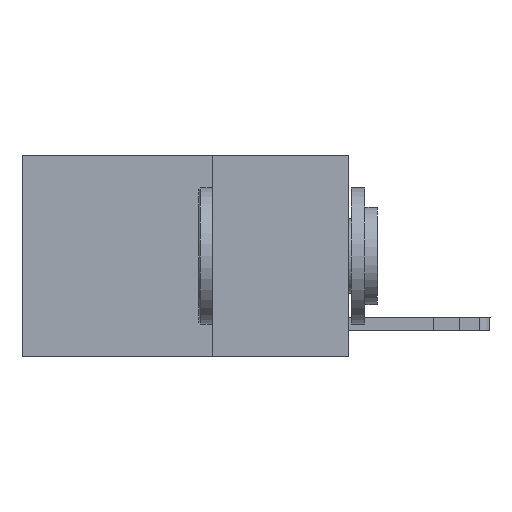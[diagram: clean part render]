
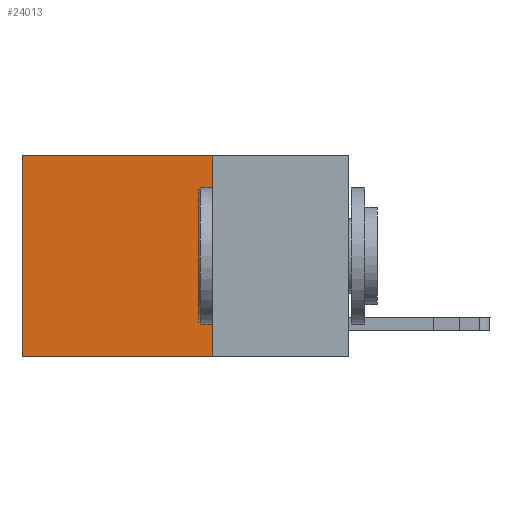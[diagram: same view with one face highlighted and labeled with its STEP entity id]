
A CAD part, left-side view. The second image highlights one B-rep face of the part: STEP entity #24013.
In plain terms, the highlighted planar face has unit normal (-1, 0, 0).
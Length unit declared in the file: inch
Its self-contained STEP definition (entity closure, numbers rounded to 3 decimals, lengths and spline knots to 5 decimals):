
#154 = LINE ( 'NONE', #15666, #4156 ) ;
#2288 = CARTESIAN_POINT ( 'NONE',  ( 0.2625, 0.6, 0. ) ) ;
#2876 = AXIS2_PLACEMENT_3D ( 'NONE', #24918, #23060, #11424 ) ;
#3390 = LINE ( 'NONE', #8488, #9211 ) ;
#3895 = CARTESIAN_POINT ( 'NONE',  ( 0.2625, 0.6, 0. ) ) ;
#4156 = VECTOR ( 'NONE', #19474, 39.37008 ) ;
#4313 = VERTEX_POINT ( 'NONE', #13982 ) ;
#4342 = VERTEX_POINT ( 'NONE', #6305 ) ;
#5892 = DIRECTION ( 'NONE',  ( 0., 0., -1. ) ) ;
#6305 = CARTESIAN_POINT ( 'NONE',  ( 0.2625, 0.25, 0. ) ) ;
#6388 = VECTOR ( 'NONE', #18502, 39.37008 ) ;
#7095 = EDGE_CURVE ( 'NONE', #4342, #11308, #154, .T. ) ;
#8488 = CARTESIAN_POINT ( 'NONE',  ( 0.2625, 0.25, 0. ) ) ;
#8489 = LINE ( 'NONE', #3895, #13021 ) ;
#8860 = CARTESIAN_POINT ( 'NONE',  ( 0.2625, 0.25, -0.37 ) ) ;
#9211 = VECTOR ( 'NONE', #12383, 39.37008 ) ;
#9719 = EDGE_CURVE ( 'NONE', #4313, #21004, #11522, .T. ) ;
#9851 = ORIENTED_EDGE ( 'NONE', *, *, #7095, .T. ) ;
#9895 = EDGE_CURVE ( 'NONE', #11308, #21004, #8489, .T. ) ;
#11308 = VERTEX_POINT ( 'NONE', #2288 ) ;
#11424 = DIRECTION ( 'NONE',  ( 0., 0., -1. ) ) ;
#11522 = LINE ( 'NONE', #8860, #6388 ) ;
#11846 = ORIENTED_EDGE ( 'NONE', *, *, #9895, .T. ) ;
#12383 = DIRECTION ( 'NONE',  ( 0., 0., -1. ) ) ;
#12443 = FACE_OUTER_BOUND ( 'NONE', #15029, .T. ) ;
#13021 = VECTOR ( 'NONE', #5892, 39.37008 ) ;
#13982 = CARTESIAN_POINT ( 'NONE',  ( 0.2625, 0.25, -0.37 ) ) ;
#15029 = EDGE_LOOP ( 'NONE', ( #11846, #23414, #19844, #9851 ) ) ;
#15666 = CARTESIAN_POINT ( 'NONE',  ( 0.2625, 0.25, 0. ) ) ;
#15995 = CARTESIAN_POINT ( 'NONE',  ( 0.2625, 0.6, -0.37 ) ) ;
#18502 = DIRECTION ( 'NONE',  ( 0., 1., 0. ) ) ;
#19116 = PLANE ( 'NONE',  #2876 ) ;
#19474 = DIRECTION ( 'NONE',  ( 0., 1., 0. ) ) ;
#19844 = ORIENTED_EDGE ( 'NONE', *, *, #22226, .F. ) ;
#21004 = VERTEX_POINT ( 'NONE', #15995 ) ;
#22226 = EDGE_CURVE ( 'NONE', #4342, #4313, #3390, .T. ) ;
#23060 = DIRECTION ( 'NONE',  ( 1., 0., 0. ) ) ;
#23414 = ORIENTED_EDGE ( 'NONE', *, *, #9719, .F. ) ;
#24013 = ADVANCED_FACE ( 'NONE', ( #12443 ), #19116, .F. ) ;
#24918 = CARTESIAN_POINT ( 'NONE',  ( 0.2625, 0.25, 0. ) ) ;
